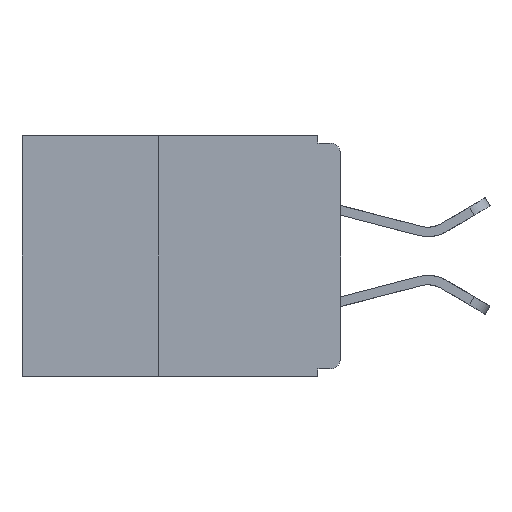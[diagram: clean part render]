
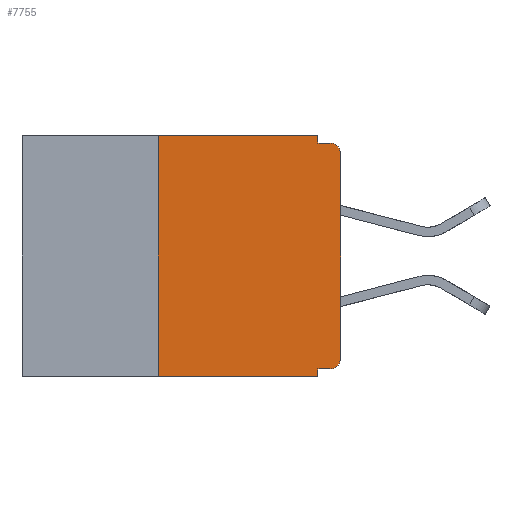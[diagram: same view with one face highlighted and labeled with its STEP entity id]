
A CAD part, left-side view. The second image highlights one B-rep face of the part: STEP entity #7755.
In plain terms, the highlighted planar face has unit normal (-1, 0, 0).
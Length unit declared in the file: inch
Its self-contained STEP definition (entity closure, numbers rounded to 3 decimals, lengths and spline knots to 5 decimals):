
#111 = AXIS2_PLACEMENT_3D ( 'NONE', #14105, #11841, #16403 ) ;
#572 = CARTESIAN_POINT ( 'NONE',  ( 0., 0.015, -0.305 ) ) ;
#874 = EDGE_CURVE ( 'NONE', #29640, #10760, #947, .T. ) ;
#947 = CIRCLE ( 'NONE', #11667, 0.015 ) ;
#1023 = VECTOR ( 'NONE', #22684, 39.37008 ) ;
#1619 = CIRCLE ( 'NONE', #18659, 0.015 ) ;
#2219 = EDGE_CURVE ( 'NONE', #22706, #14285, #1619, .T. ) ;
#2513 = EDGE_CURVE ( 'NONE', #2562, #15219, #23167, .T. ) ;
#2562 = VERTEX_POINT ( 'NONE', #16424 ) ;
#2637 = EDGE_LOOP ( 'NONE', ( #10284, #17141, #19320, #7749, #21930, #28059, #20086, #11087, #29490, #16120 ) ) ;
#3269 = CARTESIAN_POINT ( 'NONE',  ( 0., 0.25, -0.33 ) ) ;
#3271 = VERTEX_POINT ( 'NONE', #15972 ) ;
#3495 = EDGE_CURVE ( 'NONE', #12600, #18957, #28498, .T. ) ;
#3694 = CARTESIAN_POINT ( 'NONE',  ( 0., 0.031, -0.33 ) ) ;
#3896 = CARTESIAN_POINT ( 'NONE',  ( 0., 0., -0.32 ) ) ;
#4680 = DIRECTION ( 'NONE',  ( 0., -1., 0. ) ) ;
#4700 = CARTESIAN_POINT ( 'NONE',  ( 0., 0.031, -0.33 ) ) ;
#5471 = CARTESIAN_POINT ( 'NONE',  ( 0., 0.015, -0.01 ) ) ;
#5619 = CARTESIAN_POINT ( 'NONE',  ( 0., 0.437, -0.33 ) ) ;
#5706 = DIRECTION ( 'NONE',  ( 0., 0., 1. ) ) ;
#6607 = LINE ( 'NONE', #22380, #23663 ) ;
#7749 = ORIENTED_EDGE ( 'NONE', *, *, #10189, .F. ) ;
#7755 = ADVANCED_FACE ( 'NONE', ( #29626 ), #18645, .F. ) ;
#7925 = VECTOR ( 'NONE', #5706, 39.37008 ) ;
#8117 = LINE ( 'NONE', #24916, #1023 ) ;
#8452 = LINE ( 'NONE', #3896, #27678 ) ;
#8814 = DIRECTION ( 'NONE',  ( -1., 0., 0. ) ) ;
#8902 = DIRECTION ( 'NONE',  ( 0., 0., -1. ) ) ;
#8978 = CARTESIAN_POINT ( 'NONE',  ( 0., 0.015, -0.32 ) ) ;
#9439 = DIRECTION ( 'NONE',  ( 0., 0., -1. ) ) ;
#10189 = EDGE_CURVE ( 'NONE', #18957, #18902, #6607, .T. ) ;
#10284 = ORIENTED_EDGE ( 'NONE', *, *, #15691, .T. ) ;
#10489 = DIRECTION ( 'NONE',  ( -1., 0., 0. ) ) ;
#10760 = VERTEX_POINT ( 'NONE', #12893 ) ;
#11087 = ORIENTED_EDGE ( 'NONE', *, *, #16273, .F. ) ;
#11667 = AXIS2_PLACEMENT_3D ( 'NONE', #572, #10489, #9439 ) ;
#11841 = DIRECTION ( 'NONE',  ( 1., 0., 0. ) ) ;
#12600 = VERTEX_POINT ( 'NONE', #24435 ) ;
#12893 = CARTESIAN_POINT ( 'NONE',  ( 0., 0., -0.305 ) ) ;
#14105 = CARTESIAN_POINT ( 'NONE',  ( 0., 0.437, 0. ) ) ;
#14285 = VERTEX_POINT ( 'NONE', #5471 ) ;
#15219 = VERTEX_POINT ( 'NONE', #4700 ) ;
#15452 = VECTOR ( 'NONE', #24586, 39.37008 ) ;
#15691 = EDGE_CURVE ( 'NONE', #10760, #22706, #8117, .T. ) ;
#15972 = CARTESIAN_POINT ( 'NONE',  ( 0., 0.031, -0.32 ) ) ;
#16120 = ORIENTED_EDGE ( 'NONE', *, *, #874, .T. ) ;
#16273 = EDGE_CURVE ( 'NONE', #3271, #15219, #24120, .T. ) ;
#16403 = DIRECTION ( 'NONE',  ( 0., 0., -1. ) ) ;
#16424 = CARTESIAN_POINT ( 'NONE',  ( 0., 0.25, -0.33 ) ) ;
#17141 = ORIENTED_EDGE ( 'NONE', *, *, #2219, .T. ) ;
#17674 = DIRECTION ( 'NONE',  ( 0., 0., -1. ) ) ;
#17701 = VECTOR ( 'NONE', #26947, 39.37008 ) ;
#18604 = CARTESIAN_POINT ( 'NONE',  ( 0., 0., -0.01 ) ) ;
#18645 = PLANE ( 'NONE',  #111 ) ;
#18659 = AXIS2_PLACEMENT_3D ( 'NONE', #22609, #8814, #8902 ) ;
#18902 = VERTEX_POINT ( 'NONE', #26617 ) ;
#18957 = VERTEX_POINT ( 'NONE', #22252 ) ;
#18997 = CARTESIAN_POINT ( 'NONE',  ( 0., 0.437, 0. ) ) ;
#19320 = ORIENTED_EDGE ( 'NONE', *, *, #26972, .F. ) ;
#20086 = ORIENTED_EDGE ( 'NONE', *, *, #2513, .T. ) ;
#20169 = DIRECTION ( 'NONE',  ( 0., 1., 0. ) ) ;
#20713 = EDGE_CURVE ( 'NONE', #2562, #12600, #26433, .T. ) ;
#21305 = CARTESIAN_POINT ( 'NONE',  ( 0., 0., -0.025 ) ) ;
#21647 = VECTOR ( 'NONE', #4680, 39.37008 ) ;
#21930 = ORIENTED_EDGE ( 'NONE', *, *, #3495, .F. ) ;
#22252 = CARTESIAN_POINT ( 'NONE',  ( 0., 0.031, 0. ) ) ;
#22375 = LINE ( 'NONE', #18604, #21647 ) ;
#22380 = CARTESIAN_POINT ( 'NONE',  ( 0., 0.031, 0. ) ) ;
#22609 = CARTESIAN_POINT ( 'NONE',  ( 0., 0.015, -0.025 ) ) ;
#22684 = DIRECTION ( 'NONE',  ( 0., 0., 1. ) ) ;
#22706 = VERTEX_POINT ( 'NONE', #21305 ) ;
#23167 = LINE ( 'NONE', #5619, #17701 ) ;
#23382 = VECTOR ( 'NONE', #27015, 39.37008 ) ;
#23663 = VECTOR ( 'NONE', #17674, 39.37008 ) ;
#24120 = LINE ( 'NONE', #3694, #23382 ) ;
#24435 = CARTESIAN_POINT ( 'NONE',  ( 0., 0.25, 0. ) ) ;
#24586 = DIRECTION ( 'NONE',  ( 0., -1., 0. ) ) ;
#24916 = CARTESIAN_POINT ( 'NONE',  ( 0., 0., 0. ) ) ;
#26433 = LINE ( 'NONE', #3269, #7925 ) ;
#26617 = CARTESIAN_POINT ( 'NONE',  ( 0., 0.031, -0.01 ) ) ;
#26947 = DIRECTION ( 'NONE',  ( 0., -1., 0. ) ) ;
#26972 = EDGE_CURVE ( 'NONE', #18902, #14285, #22375, .T. ) ;
#27015 = DIRECTION ( 'NONE',  ( 0., 0., -1. ) ) ;
#27678 = VECTOR ( 'NONE', #20169, 39.37008 ) ;
#28059 = ORIENTED_EDGE ( 'NONE', *, *, #20713, .F. ) ;
#28498 = LINE ( 'NONE', #18997, #15452 ) ;
#29490 = ORIENTED_EDGE ( 'NONE', *, *, #30140, .F. ) ;
#29626 = FACE_OUTER_BOUND ( 'NONE', #2637, .T. ) ;
#29640 = VERTEX_POINT ( 'NONE', #8978 ) ;
#30140 = EDGE_CURVE ( 'NONE', #29640, #3271, #8452, .T. ) ;
